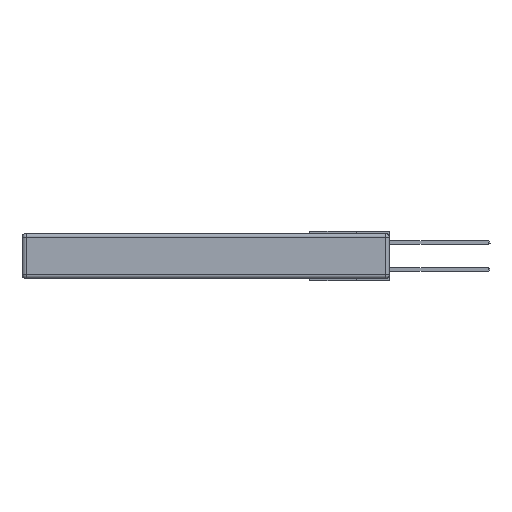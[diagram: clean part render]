
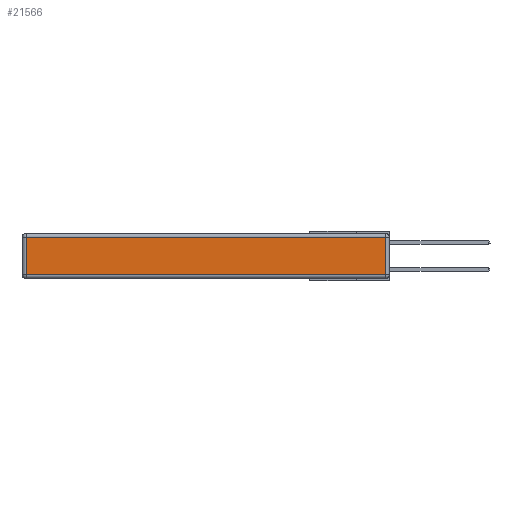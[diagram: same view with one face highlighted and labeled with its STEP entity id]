
A CAD part, left-side view. The second image highlights one B-rep face of the part: STEP entity #21566.
In plain terms, the highlighted planar face has unit normal (-1, 0, 0).
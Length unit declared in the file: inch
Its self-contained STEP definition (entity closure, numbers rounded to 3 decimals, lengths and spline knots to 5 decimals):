
#70 = AXIS2_PLACEMENT_3D ( 'NONE', #23367, #23237, #34016 ) ;
#1858 = VERTEX_POINT ( 'NONE', #18981 ) ;
#3789 = CARTESIAN_POINT ( 'NONE',  ( 0., 2.72, -0.03 ) ) ;
#4300 = DIRECTION ( 'NONE',  ( 0., -1., 0. ) ) ;
#5477 = CARTESIAN_POINT ( 'NONE',  ( 0., 0.03, -0.313 ) ) ;
#5508 = FACE_OUTER_BOUND ( 'NONE', #28190, .T. ) ;
#6652 = EDGE_CURVE ( 'NONE', #27172, #1858, #11711, .T. ) ;
#7458 = CARTESIAN_POINT ( 'NONE',  ( 0., 2.75, -0.03 ) ) ;
#10205 = ORIENTED_EDGE ( 'NONE', *, *, #22717, .T. ) ;
#10644 = DIRECTION ( 'NONE',  ( 0., 0., 1. ) ) ;
#11711 = LINE ( 'NONE', #19663, #30013 ) ;
#12445 = CARTESIAN_POINT ( 'NONE',  ( 0., 0., -0.313 ) ) ;
#12985 = DIRECTION ( 'NONE',  ( 0., 1., 0. ) ) ;
#14908 = EDGE_CURVE ( 'NONE', #20038, #21249, #28058, .T. ) ;
#15910 = ORIENTED_EDGE ( 'NONE', *, *, #6652, .T. ) ;
#16206 = VECTOR ( 'NONE', #12985, 39.37008 ) ;
#18138 = VECTOR ( 'NONE', #4300, 39.37008 ) ;
#18981 = CARTESIAN_POINT ( 'NONE',  ( 0., 0.03, -0.03 ) ) ;
#19663 = CARTESIAN_POINT ( 'NONE',  ( 0., 0.03, -0.343 ) ) ;
#20038 = VERTEX_POINT ( 'NONE', #3789 ) ;
#20304 = EDGE_CURVE ( 'NONE', #1858, #20038, #23902, .T. ) ;
#21249 = VERTEX_POINT ( 'NONE', #25261 ) ;
#21566 = ADVANCED_FACE ( 'NONE', ( #5508 ), #23008, .T. ) ;
#22717 = EDGE_CURVE ( 'NONE', #21249, #27172, #24124, .T. ) ;
#23008 = PLANE ( 'NONE',  #70 ) ;
#23237 = DIRECTION ( 'NONE',  ( -1., 0., 0. ) ) ;
#23367 = CARTESIAN_POINT ( 'NONE',  ( 0., 0., -0.343 ) ) ;
#23902 = LINE ( 'NONE', #7458, #16206 ) ;
#24124 = LINE ( 'NONE', #12445, #18138 ) ;
#25261 = CARTESIAN_POINT ( 'NONE',  ( 0., 2.72, -0.313 ) ) ;
#25560 = CARTESIAN_POINT ( 'NONE',  ( 0., 2.72, -0.343 ) ) ;
#26767 = ORIENTED_EDGE ( 'NONE', *, *, #20304, .T. ) ;
#27172 = VERTEX_POINT ( 'NONE', #5477 ) ;
#28058 = LINE ( 'NONE', #25560, #31482 ) ;
#28190 = EDGE_LOOP ( 'NONE', ( #10205, #15910, #26767, #34901 ) ) ;
#30013 = VECTOR ( 'NONE', #10644, 39.37008 ) ;
#30931 = DIRECTION ( 'NONE',  ( 0., 0., -1. ) ) ;
#31482 = VECTOR ( 'NONE', #30931, 39.37008 ) ;
#34016 = DIRECTION ( 'NONE',  ( 0., 0., 1. ) ) ;
#34901 = ORIENTED_EDGE ( 'NONE', *, *, #14908, .T. ) ;
